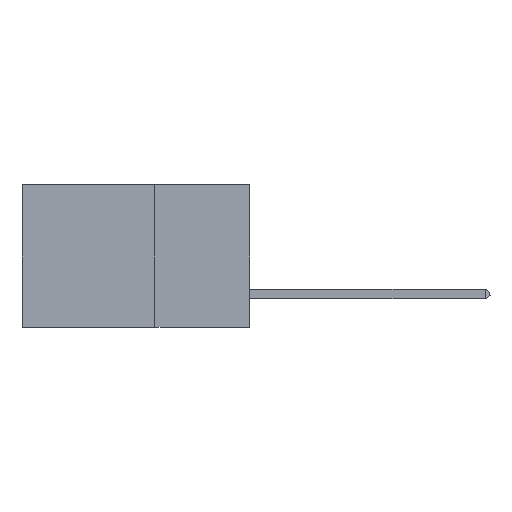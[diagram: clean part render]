
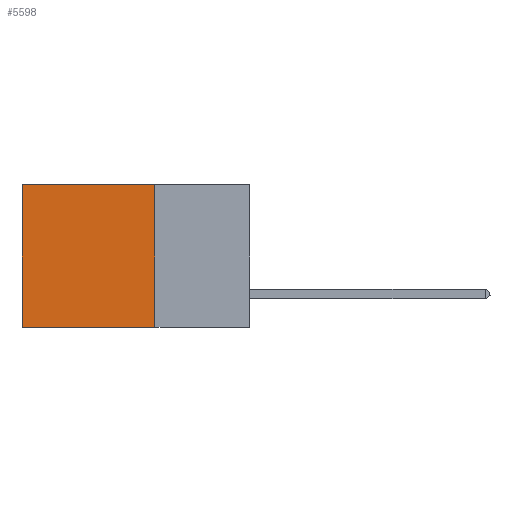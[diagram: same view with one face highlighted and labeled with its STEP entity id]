
A CAD part, left-side view. The second image highlights one B-rep face of the part: STEP entity #5598.
In plain terms, the highlighted planar face has unit normal (-1, 0, 0).
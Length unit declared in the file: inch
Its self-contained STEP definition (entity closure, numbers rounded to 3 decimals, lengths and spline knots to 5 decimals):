
#415 = DIRECTION ( 'NONE',  ( 0., 0., -1. ) ) ;
#479 = EDGE_CURVE ( 'NONE', #3874, #8270, #15401, .T. ) ;
#846 = VERTEX_POINT ( 'NONE', #8094 ) ;
#1189 = AXIS2_PLACEMENT_3D ( 'NONE', #9314, #1656, #415 ) ;
#1642 = EDGE_CURVE ( 'NONE', #8270, #6071, #5299, .T. ) ;
#1656 = DIRECTION ( 'NONE',  ( 1., 0., 0. ) ) ;
#1965 = VECTOR ( 'NONE', #3382, 39.37008 ) ;
#1968 = CARTESIAN_POINT ( 'NONE',  ( 0.2875, 0.6, -0.375 ) ) ;
#2102 = FACE_OUTER_BOUND ( 'NONE', #15638, .T. ) ;
#2120 = CARTESIAN_POINT ( 'NONE',  ( 0.2875, 0.25, 0. ) ) ;
#2288 = DIRECTION ( 'NONE',  ( 0., 1., 0. ) ) ;
#3382 = DIRECTION ( 'NONE',  ( 0., 0., -1. ) ) ;
#3839 = ORIENTED_EDGE ( 'NONE', *, *, #479, .T. ) ;
#3874 = VERTEX_POINT ( 'NONE', #2120 ) ;
#4874 = CARTESIAN_POINT ( 'NONE',  ( 0.2875, 0.25, -0.375 ) ) ;
#5105 = EDGE_CURVE ( 'NONE', #846, #6071, #11596, .T. ) ;
#5299 = LINE ( 'NONE', #11073, #1965 ) ;
#5598 = ADVANCED_FACE ( 'NONE', ( #2102 ), #5624, .F. ) ;
#5624 = PLANE ( 'NONE',  #1189 ) ;
#6071 = VERTEX_POINT ( 'NONE', #1968 ) ;
#6553 = CARTESIAN_POINT ( 'NONE',  ( 0.2875, 0.25, -0.375 ) ) ;
#6685 = ORIENTED_EDGE ( 'NONE', *, *, #12064, .F. ) ;
#7487 = VECTOR ( 'NONE', #2288, 39.37008 ) ;
#8094 = CARTESIAN_POINT ( 'NONE',  ( 0.2875, 0.25, -0.375 ) ) ;
#8270 = VERTEX_POINT ( 'NONE', #11611 ) ;
#8771 = VECTOR ( 'NONE', #13499, 39.37008 ) ;
#9047 = VECTOR ( 'NONE', #15127, 39.37008 ) ;
#9314 = CARTESIAN_POINT ( 'NONE',  ( 0.2875, 0.25, -0.375 ) ) ;
#9687 = ORIENTED_EDGE ( 'NONE', *, *, #1642, .T. ) ;
#11073 = CARTESIAN_POINT ( 'NONE',  ( 0.2875, 0.6, -0.375 ) ) ;
#11596 = LINE ( 'NONE', #4874, #7487 ) ;
#11611 = CARTESIAN_POINT ( 'NONE',  ( 0.2875, 0.6, 0. ) ) ;
#12064 = EDGE_CURVE ( 'NONE', #3874, #846, #12373, .T. ) ;
#12373 = LINE ( 'NONE', #6553, #9047 ) ;
#13499 = DIRECTION ( 'NONE',  ( 0., 1., 0. ) ) ;
#15127 = DIRECTION ( 'NONE',  ( 0., 0., -1. ) ) ;
#15401 = LINE ( 'NONE', #16009, #8771 ) ;
#15625 = ORIENTED_EDGE ( 'NONE', *, *, #5105, .F. ) ;
#15638 = EDGE_LOOP ( 'NONE', ( #9687, #15625, #6685, #3839 ) ) ;
#16009 = CARTESIAN_POINT ( 'NONE',  ( 0.2875, 0.25, 0. ) ) ;
